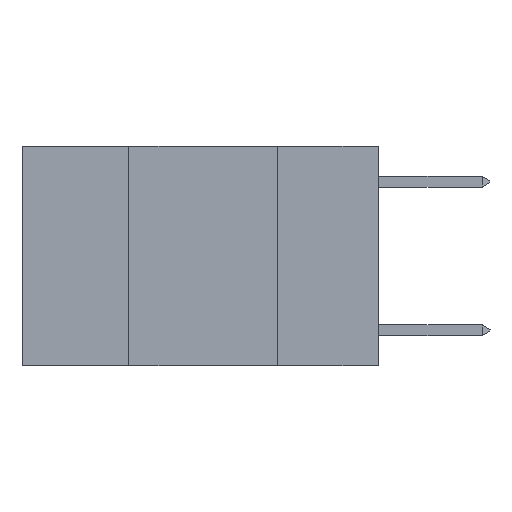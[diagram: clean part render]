
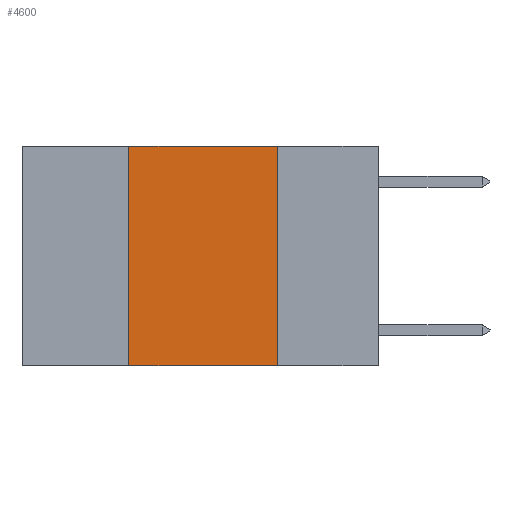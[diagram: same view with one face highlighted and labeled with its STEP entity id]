
A CAD part, left-side view. The second image highlights one B-rep face of the part: STEP entity #4600.
In plain terms, the highlighted planar face has unit normal (-1, 0, 0).
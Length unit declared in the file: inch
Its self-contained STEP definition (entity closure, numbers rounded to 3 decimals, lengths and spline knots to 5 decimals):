
#1157 = ORIENTED_EDGE ( 'NONE', *, *, #6597, .F. ) ;
#1320 = EDGE_CURVE ( 'NONE', #18034, #14249, #23151, .T. ) ;
#2672 = EDGE_CURVE ( 'NONE', #18034, #5582, #14596, .T. ) ;
#3594 = VERTEX_POINT ( 'NONE', #16065 ) ;
#3788 = CARTESIAN_POINT ( 'NONE',  ( 0., 0.42, 0. ) ) ;
#4228 = AXIS2_PLACEMENT_3D ( 'NONE', #22147, #22003, #21982 ) ;
#4301 = DIRECTION ( 'NONE',  ( 0., 0., 1. ) ) ;
#4600 = ADVANCED_FACE ( 'NONE', ( #16404 ), #22079, .F. ) ;
#5582 = VERTEX_POINT ( 'NONE', #16282 ) ;
#6597 = EDGE_CURVE ( 'NONE', #3594, #14249, #15337, .T. ) ;
#7143 = CARTESIAN_POINT ( 'NONE',  ( 0., 0.6, -0.37 ) ) ;
#10584 = EDGE_CURVE ( 'NONE', #5582, #3594, #18499, .T. ) ;
#11476 = VECTOR ( 'NONE', #18604, 39.37008 ) ;
#14249 = VERTEX_POINT ( 'NONE', #21525 ) ;
#14412 = VECTOR ( 'NONE', #4301, 39.37008 ) ;
#14596 = LINE ( 'NONE', #3788, #14412 ) ;
#15337 = LINE ( 'NONE', #18929, #11476 ) ;
#15552 = EDGE_LOOP ( 'NONE', ( #1157, #18535, #22986, #22858 ) ) ;
#16065 = CARTESIAN_POINT ( 'NONE',  ( 0., 0.17, 0. ) ) ;
#16282 = CARTESIAN_POINT ( 'NONE',  ( 0., 0.42, 0. ) ) ;
#16404 = FACE_OUTER_BOUND ( 'NONE', #15552, .T. ) ;
#18034 = VERTEX_POINT ( 'NONE', #21014 ) ;
#18173 = VECTOR ( 'NONE', #20030, 39.37008 ) ;
#18499 = LINE ( 'NONE', #20077, #18173 ) ;
#18535 = ORIENTED_EDGE ( 'NONE', *, *, #10584, .F. ) ;
#18604 = DIRECTION ( 'NONE',  ( 0., 0., -1. ) ) ;
#18929 = CARTESIAN_POINT ( 'NONE',  ( 0., 0.17, 0. ) ) ;
#20030 = DIRECTION ( 'NONE',  ( 0., -1., 0. ) ) ;
#20077 = CARTESIAN_POINT ( 'NONE',  ( 0., 0.6, 0. ) ) ;
#21014 = CARTESIAN_POINT ( 'NONE',  ( 0., 0.42, -0.37 ) ) ;
#21525 = CARTESIAN_POINT ( 'NONE',  ( 0., 0.17, -0.37 ) ) ;
#21982 = DIRECTION ( 'NONE',  ( 0., 0., -1. ) ) ;
#22003 = DIRECTION ( 'NONE',  ( 1., 0., 0. ) ) ;
#22079 = PLANE ( 'NONE',  #4228 ) ;
#22147 = CARTESIAN_POINT ( 'NONE',  ( 0., 0.6, 0. ) ) ;
#22630 = VECTOR ( 'NONE', #24104, 39.37008 ) ;
#22858 = ORIENTED_EDGE ( 'NONE', *, *, #1320, .T. ) ;
#22986 = ORIENTED_EDGE ( 'NONE', *, *, #2672, .F. ) ;
#23151 = LINE ( 'NONE', #7143, #22630 ) ;
#24104 = DIRECTION ( 'NONE',  ( 0., -1., 0. ) ) ;
